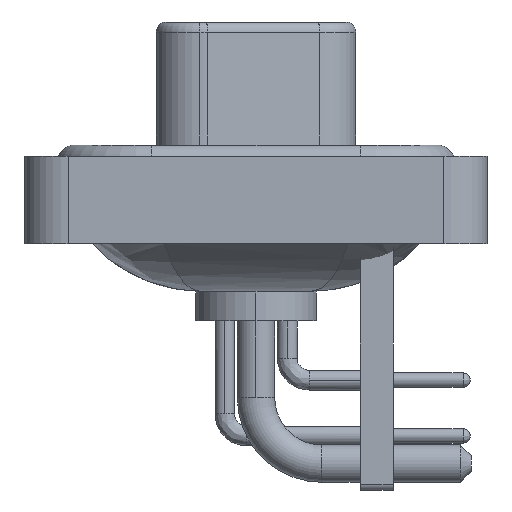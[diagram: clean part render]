
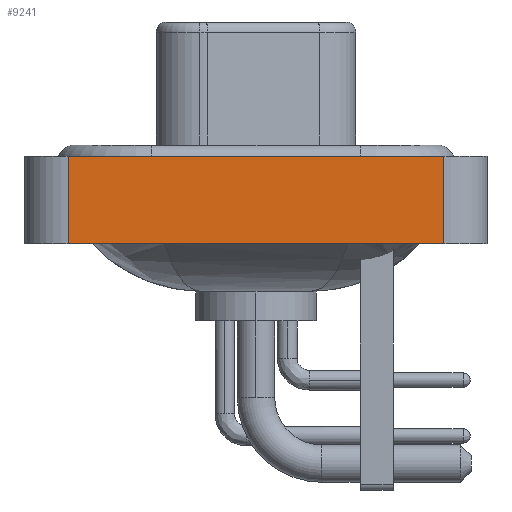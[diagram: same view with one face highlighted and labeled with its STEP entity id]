
A CAD part, left-side view. The second image highlights one B-rep face of the part: STEP entity #9241.
In plain terms, the highlighted planar face has unit normal (-1, 0, 0).
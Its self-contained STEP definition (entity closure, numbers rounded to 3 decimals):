
#321 = VERTEX_POINT ( 'NONE', #12740 ) ;
#1371 = LINE ( 'NONE', #9777, #21798 ) ;
#3423 = LINE ( 'NONE', #15904, #23379 ) ;
#3595 = VECTOR ( 'NONE', #24047, 1000. ) ;
#5054 = EDGE_CURVE ( 'NONE', #9706, #321, #9887, .T. ) ;
#5589 = DIRECTION ( 'NONE',  ( 0., 0., 1. ) ) ;
#6806 = FACE_OUTER_BOUND ( 'NONE', #26401, .T. ) ;
#7319 = LINE ( 'NONE', #15867, #3595 ) ;
#7844 = ORIENTED_EDGE ( 'NONE', *, *, #18417, .T. ) ;
#7990 = ORIENTED_EDGE ( 'NONE', *, *, #5054, .T. ) ;
#8296 = CARTESIAN_POINT ( 'NONE',  ( -7.35, 8.55, -3.6 ) ) ;
#8812 = CARTESIAN_POINT ( 'NONE',  ( -7.35, 8.55, 0.4 ) ) ;
#9241 = ADVANCED_FACE ( 'NONE', ( #6806 ), #17398, .T. ) ;
#9395 = VERTEX_POINT ( 'NONE', #8296 ) ;
#9655 = DIRECTION ( 'NONE',  ( 0., -1., 0. ) ) ;
#9706 = VERTEX_POINT ( 'NONE', #16976 ) ;
#9777 = CARTESIAN_POINT ( 'NONE',  ( -7.35, -8.55, -3.6 ) ) ;
#9887 = LINE ( 'NONE', #24865, #18747 ) ;
#10131 = ORIENTED_EDGE ( 'NONE', *, *, #15349, .F. ) ;
#12645 = AXIS2_PLACEMENT_3D ( 'NONE', #15093, #13039, #25724 ) ;
#12740 = CARTESIAN_POINT ( 'NONE',  ( -7.35, -8.55, 0.4 ) ) ;
#13039 = DIRECTION ( 'NONE',  ( -1., 0., 0. ) ) ;
#15093 = CARTESIAN_POINT ( 'NONE',  ( -7.35, -8.55, -3.6 ) ) ;
#15349 = EDGE_CURVE ( 'NONE', #9395, #23017, #3423, .T. ) ;
#15867 = CARTESIAN_POINT ( 'NONE',  ( -7.35, -8.55, 0.4 ) ) ;
#15904 = CARTESIAN_POINT ( 'NONE',  ( -7.35, 8.55, -3.6 ) ) ;
#16976 = CARTESIAN_POINT ( 'NONE',  ( -7.35, -8.55, -3.6 ) ) ;
#17398 = PLANE ( 'NONE',  #12645 ) ;
#18417 = EDGE_CURVE ( 'NONE', #9395, #9706, #1371, .T. ) ;
#18747 = VECTOR ( 'NONE', #26642, 1000. ) ;
#21372 = ORIENTED_EDGE ( 'NONE', *, *, #26882, .F. ) ;
#21798 = VECTOR ( 'NONE', #9655, 1000. ) ;
#23017 = VERTEX_POINT ( 'NONE', #8812 ) ;
#23379 = VECTOR ( 'NONE', #5589, 1000. ) ;
#24047 = DIRECTION ( 'NONE',  ( 0., -1., 0. ) ) ;
#24865 = CARTESIAN_POINT ( 'NONE',  ( -7.35, -8.55, -3.6 ) ) ;
#25724 = DIRECTION ( 'NONE',  ( 0., 0., 1. ) ) ;
#26401 = EDGE_LOOP ( 'NONE', ( #7990, #21372, #10131, #7844 ) ) ;
#26642 = DIRECTION ( 'NONE',  ( 0., 0., 1. ) ) ;
#26882 = EDGE_CURVE ( 'NONE', #23017, #321, #7319, .T. ) ;
